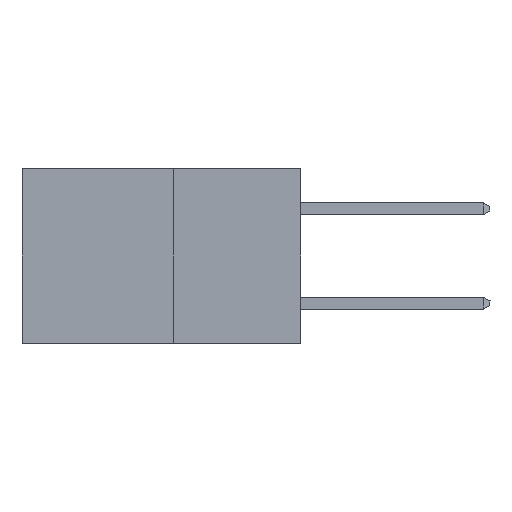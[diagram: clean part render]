
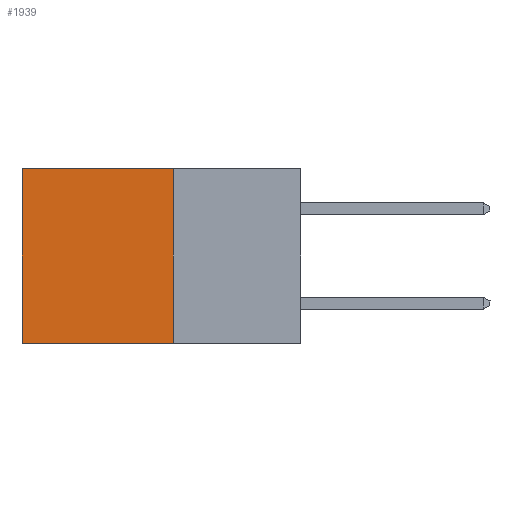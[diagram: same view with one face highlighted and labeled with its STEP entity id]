
A CAD part, left-side view. The second image highlights one B-rep face of the part: STEP entity #1939.
In plain terms, the highlighted planar face has unit normal (-1, 0, 0).
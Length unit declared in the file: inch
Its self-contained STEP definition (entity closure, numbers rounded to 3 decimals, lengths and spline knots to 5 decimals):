
#184 = CARTESIAN_POINT ( 'NONE',  ( 0.277, 0.27, -0.37 ) ) ;
#1001 = ORIENTED_EDGE ( 'NONE', *, *, #1311, .T. ) ;
#1108 = VERTEX_POINT ( 'NONE', #3681 ) ;
#1112 = EDGE_CURVE ( 'NONE', #3766, #5196, #5462, .T. ) ;
#1240 = VECTOR ( 'NONE', #8826, 39.37008 ) ;
#1311 = EDGE_CURVE ( 'NONE', #5196, #6227, #7119, .T. ) ;
#1414 = ORIENTED_EDGE ( 'NONE', *, *, #4581, .F. ) ;
#1460 = ORIENTED_EDGE ( 'NONE', *, *, #5784, .F. ) ;
#1505 = ORIENTED_EDGE ( 'NONE', *, *, #1112, .T. ) ;
#1939 = ADVANCED_FACE ( 'NONE', ( #9621 ), #2904, .F. ) ;
#2839 = DIRECTION ( 'NONE',  ( 0., 0., -1. ) ) ;
#2850 = DIRECTION ( 'NONE',  ( 1., 0., 0. ) ) ;
#2880 = CARTESIAN_POINT ( 'NONE',  ( 0.277, 0.27, -0.37 ) ) ;
#2904 = PLANE ( 'NONE',  #6848 ) ;
#2994 = CARTESIAN_POINT ( 'NONE',  ( 0.277, 0.27, 0. ) ) ;
#3052 = DIRECTION ( 'NONE',  ( 0., 1., 0. ) ) ;
#3146 = VECTOR ( 'NONE', #9573, 39.37008 ) ;
#3681 = CARTESIAN_POINT ( 'NONE',  ( 0.277, 0.27, -0.37 ) ) ;
#3766 = VERTEX_POINT ( 'NONE', #7262 ) ;
#3783 = LINE ( 'NONE', #184, #1240 ) ;
#4058 = CARTESIAN_POINT ( 'NONE',  ( 0.277, 0.59, 0. ) ) ;
#4581 = EDGE_CURVE ( 'NONE', #1108, #6227, #3783, .T. ) ;
#5196 = VERTEX_POINT ( 'NONE', #4058 ) ;
#5240 = CARTESIAN_POINT ( 'NONE',  ( 0.277, 0.59, -0.37 ) ) ;
#5462 = LINE ( 'NONE', #2994, #10554 ) ;
#5784 = EDGE_CURVE ( 'NONE', #3766, #1108, #7653, .T. ) ;
#6227 = VERTEX_POINT ( 'NONE', #5240 ) ;
#6848 = AXIS2_PLACEMENT_3D ( 'NONE', #2880, #2850, #2839 ) ;
#7119 = LINE ( 'NONE', #9746, #9128 ) ;
#7262 = CARTESIAN_POINT ( 'NONE',  ( 0.277, 0.27, 0. ) ) ;
#7653 = LINE ( 'NONE', #9586, #3146 ) ;
#8826 = DIRECTION ( 'NONE',  ( 0., 1., 0. ) ) ;
#9128 = VECTOR ( 'NONE', #9648, 39.37008 ) ;
#9288 = EDGE_LOOP ( 'NONE', ( #1001, #1414, #1460, #1505 ) ) ;
#9573 = DIRECTION ( 'NONE',  ( 0., 0., -1. ) ) ;
#9586 = CARTESIAN_POINT ( 'NONE',  ( 0.277, 0.27, -0.37 ) ) ;
#9621 = FACE_OUTER_BOUND ( 'NONE', #9288, .T. ) ;
#9648 = DIRECTION ( 'NONE',  ( 0., 0., -1. ) ) ;
#9746 = CARTESIAN_POINT ( 'NONE',  ( 0.277, 0.59, -0.37 ) ) ;
#10554 = VECTOR ( 'NONE', #3052, 39.37008 ) ;
